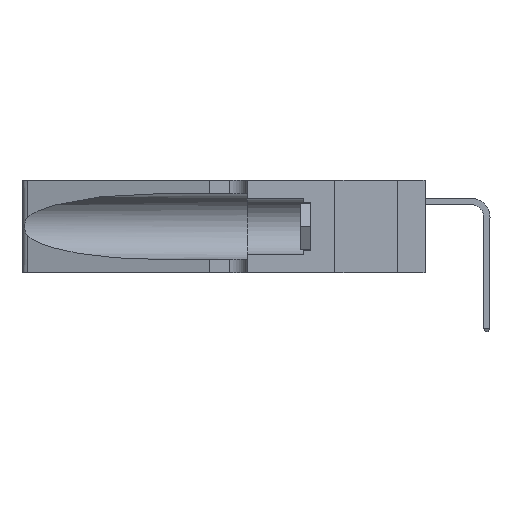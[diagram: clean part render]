
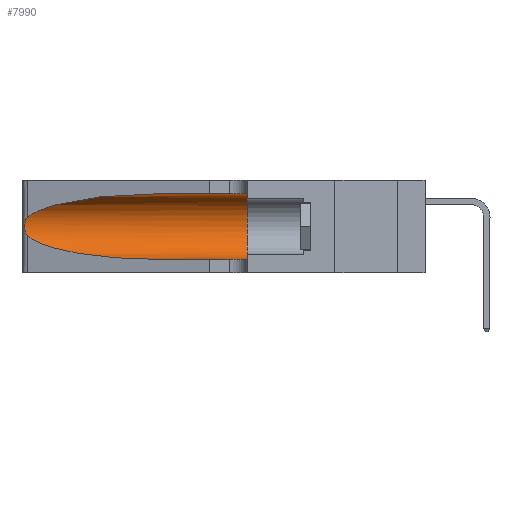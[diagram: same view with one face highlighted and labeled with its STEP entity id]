
A CAD part, left-side view. The second image highlights one B-rep face of the part: STEP entity #7990.
In plain terms, the highlighted cylindrical face has radius 3.308 mm (diameter 6.617 mm), a partial arc.
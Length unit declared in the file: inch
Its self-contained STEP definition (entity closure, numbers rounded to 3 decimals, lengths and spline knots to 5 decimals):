
#186 = CARTESIAN_POINT ( 'NONE',  ( 0.1305, 0.35, 0.185 ) ) ;
#225 = FACE_OUTER_BOUND ( 'NONE', #11792, .T. ) ;
#398 = ORIENTED_EDGE ( 'NONE', *, *, #2672, .T. ) ;
#546 = VERTEX_POINT ( 'NONE', #723 ) ;
#723 = CARTESIAN_POINT ( 'NONE',  ( 0.1305, 0.35, 0.31525 ) ) ;
#1030 = ORIENTED_EDGE ( 'NONE', *, *, #5877, .T. ) ;
#1158 = CARTESIAN_POINT ( 'NONE',  ( 0.2373, 1.15595, 0.08982 ) ) ;
#1431 = CARTESIAN_POINT ( 'NONE',  ( 0.25856, 1.23593, 0.16098 ) ) ;
#1790 = DIRECTION ( 'NONE',  ( 0., 0., 1. ) ) ;
#2053 =( BOUNDED_CURVE ( )  B_SPLINE_CURVE ( 3, ( #15321, #1158, #13812, #4366 ),
 .UNSPECIFIED., .F., .F. ) 
 B_SPLINE_CURVE_WITH_KNOTS ( ( 4, 4 ),
 ( 3.44316, 4.71239 ),
 .UNSPECIFIED. ) 
 CURVE ( )  GEOMETRIC_REPRESENTATION_ITEM ( )  RATIONAL_B_SPLINE_CURVE ( ( 1., 0.87, 0.87, 1. ) ) 
 REPRESENTATION_ITEM ( '' )  );
#2645 = CARTESIAN_POINT ( 'NONE',  ( 0.1305, 0.35, 0.05475 ) ) ;
#2653 = CARTESIAN_POINT ( 'NONE',  ( 0.25487, 1.22718, 0.14631 ) ) ;
#2672 = EDGE_CURVE ( 'NONE', #16616, #16693, #12334, .T. ) ;
#2716 = CARTESIAN_POINT ( 'NONE',  ( 0.18966, 0.96281, 0.31525 ) ) ;
#2787 = CARTESIAN_POINT ( 'NONE',  ( 0.2373, 1.15595, 0.28018 ) ) ;
#2964 = CARTESIAN_POINT ( 'NONE',  ( 0.25639, 1.23184, 0.21858 ) ) ;
#3029 = DIRECTION ( 'NONE',  ( 0., -1., 0. ) ) ;
#3034 = CARTESIAN_POINT ( 'NONE',  ( 0.25639, 1.23186, 0.15144 ) ) ;
#3646 = ORIENTED_EDGE ( 'NONE', *, *, #8180, .F. ) ;
#3967 = CYLINDRICAL_SURFACE ( 'NONE', #8718, 0.13025 ) ;
#4273 = ORIENTED_EDGE ( 'NONE', *, *, #13330, .T. ) ;
#4366 = CARTESIAN_POINT ( 'NONE',  ( 0.1305, 0.72297, 0.05475 ) ) ;
#4380 = VERTEX_POINT ( 'NONE', #19431 ) ;
#4651 = CARTESIAN_POINT ( 'NONE',  ( 0.25487, 1.22718, 0.14631 ) ) ;
#5877 = EDGE_CURVE ( 'NONE', #6371, #6366, #13066, .T. ) ;
#6366 = VERTEX_POINT ( 'NONE', #2653 ) ;
#6371 = VERTEX_POINT ( 'NONE', #16795 ) ;
#7232 = CARTESIAN_POINT ( 'NONE',  ( 0.1305, 0.72297, 0.05475 ) ) ;
#7750 = CARTESIAN_POINT ( 'NONE',  ( 0.25854, 1.2359, 0.20912 ) ) ;
#7804 = VECTOR ( 'NONE', #15806, 39.37008 ) ;
#7990 = ADVANCED_FACE ( 'NONE', ( #225 ), #3967, .F. ) ;
#8180 = EDGE_CURVE ( 'NONE', #546, #16693, #12568, .T. ) ;
#8718 = AXIS2_PLACEMENT_3D ( 'NONE', #16961, #13813, #9140 ) ;
#9140 = DIRECTION ( 'NONE',  ( 0., 0., -1. ) ) ;
#9335 = CARTESIAN_POINT ( 'NONE',  ( 0.26075, 1.23896, 0.19203 ) ) ;
#9483 = CARTESIAN_POINT ( 'NONE',  ( 0.1305, 1.61858, 0.31525 ) ) ;
#9598 = EDGE_CURVE ( 'NONE', #6366, #16616, #2053, .T. ) ;
#9635 = ORIENTED_EDGE ( 'NONE', *, *, #11537, .F. ) ;
#10897 = CARTESIAN_POINT ( 'NONE',  ( 0.26017, 1.23833, 0.17102 ) ) ;
#11252 = DIRECTION ( 'NONE',  ( 0., 1., 0. ) ) ;
#11371 = VECTOR ( 'NONE', #3029, 39.37008 ) ;
#11537 = EDGE_CURVE ( 'NONE', #4380, #546, #11964, .T. ) ;
#11763 = ORIENTED_EDGE ( 'NONE', *, *, #9598, .T. ) ;
#11792 = EDGE_LOOP ( 'NONE', ( #4273, #1030, #11763, #398, #3646, #9635 ) ) ;
#11964 = LINE ( 'NONE', #9483, #7804 ) ;
#12334 = LINE ( 'NONE', #14071, #11371 ) ;
#12468 = CARTESIAN_POINT ( 'NONE',  ( 0.25789, 1.23486, 0.15765 ) ) ;
#12568 = CIRCLE ( 'NONE', #19191, 0.13025 ) ;
#13066 = B_SPLINE_CURVE_WITH_KNOTS ( 'NONE', 3,
 ( #15582, #14007, #2964, #17149, #7750, #18695, #9335, #20262, #10897, #1431, #12468, #3034, #14074, #4651 ),
 .UNSPECIFIED., .F., .F.,
 ( 4, 2, 2, 2, 2, 2, 4 ),
 ( 0., 0.00027, 0.00053, 0.00107, 0.0016, 0.00187, 0.00214 ),
 .UNSPECIFIED. ) ;
#13330 = EDGE_CURVE ( 'NONE', #4380, #6371, #15200, .T. ) ;
#13812 = CARTESIAN_POINT ( 'NONE',  ( 0.18966, 0.96281, 0.05475 ) ) ;
#13813 = DIRECTION ( 'NONE',  ( 0., -1., 0. ) ) ;
#13838 = CARTESIAN_POINT ( 'NONE',  ( 0.25487, 1.22718, 0.22369 ) ) ;
#14007 = CARTESIAN_POINT ( 'NONE',  ( 0.25555, 1.22994, 0.2215 ) ) ;
#14071 = CARTESIAN_POINT ( 'NONE',  ( 0.1305, 1.61858, 0.05475 ) ) ;
#14074 = CARTESIAN_POINT ( 'NONE',  ( 0.25555, 1.22993, 0.14849 ) ) ;
#15200 =( BOUNDED_CURVE ( )  B_SPLINE_CURVE ( 3, ( #20028, #2716, #2787, #13838 ),
 .UNSPECIFIED., .F., .F. ) 
 B_SPLINE_CURVE_WITH_KNOTS ( ( 4, 4 ),
 ( 1.5708, 2.84003 ),
 .UNSPECIFIED. ) 
 CURVE ( )  GEOMETRIC_REPRESENTATION_ITEM ( )  RATIONAL_B_SPLINE_CURVE ( ( 1., 0.87, 0.87, 1. ) ) 
 REPRESENTATION_ITEM ( '' )  );
#15321 = CARTESIAN_POINT ( 'NONE',  ( 0.25487, 1.22718, 0.14631 ) ) ;
#15582 = CARTESIAN_POINT ( 'NONE',  ( 0.25487, 1.22718, 0.22369 ) ) ;
#15806 = DIRECTION ( 'NONE',  ( 0., -1., 0. ) ) ;
#16616 = VERTEX_POINT ( 'NONE', #7232 ) ;
#16693 = VERTEX_POINT ( 'NONE', #2645 ) ;
#16795 = CARTESIAN_POINT ( 'NONE',  ( 0.25487, 1.22718, 0.22369 ) ) ;
#16961 = CARTESIAN_POINT ( 'NONE',  ( 0.1305, 1.61858, 0.185 ) ) ;
#17149 = CARTESIAN_POINT ( 'NONE',  ( 0.25787, 1.23484, 0.2124 ) ) ;
#18695 = CARTESIAN_POINT ( 'NONE',  ( 0.26018, 1.23835, 0.19895 ) ) ;
#19191 = AXIS2_PLACEMENT_3D ( 'NONE', #186, #11252, #1790 ) ;
#19431 = CARTESIAN_POINT ( 'NONE',  ( 0.1305, 0.72297, 0.31525 ) ) ;
#20028 = CARTESIAN_POINT ( 'NONE',  ( 0.1305, 0.72297, 0.31525 ) ) ;
#20262 = CARTESIAN_POINT ( 'NONE',  ( 0.26075, 1.23896, 0.178 ) ) ;
